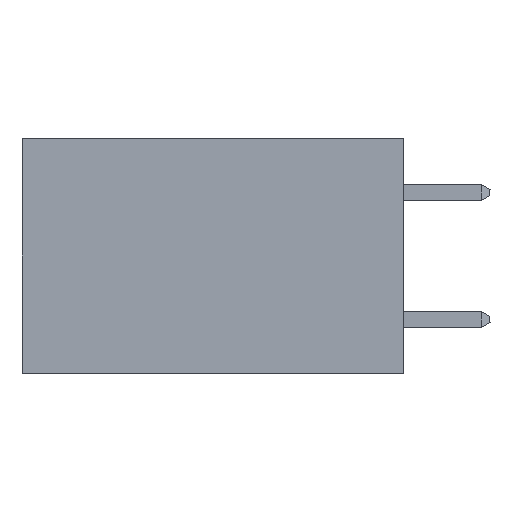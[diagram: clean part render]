
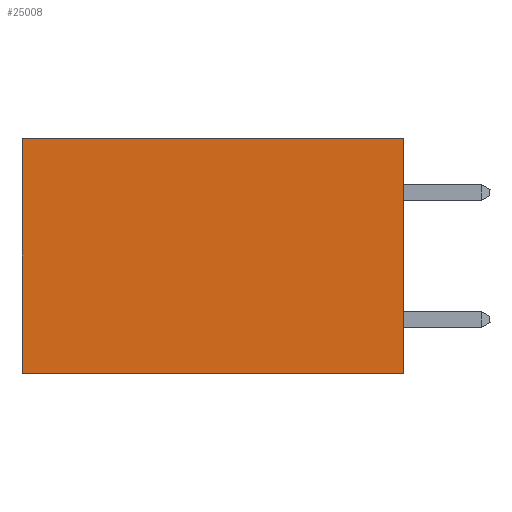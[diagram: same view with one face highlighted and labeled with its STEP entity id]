
A CAD part, left-side view. The second image highlights one B-rep face of the part: STEP entity #25008.
In plain terms, the highlighted planar face has unit normal (-1, 0, 0).
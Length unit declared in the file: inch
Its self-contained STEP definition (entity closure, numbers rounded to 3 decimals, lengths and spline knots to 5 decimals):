
#365 = VECTOR ( 'NONE', #31459, 39.37008 ) ;
#2578 = CARTESIAN_POINT ( 'NONE',  ( 0.2875, 0., -0.37 ) ) ;
#3232 = VERTEX_POINT ( 'NONE', #40267 ) ;
#3275 = ORIENTED_EDGE ( 'NONE', *, *, #23552, .F. ) ;
#4162 = CARTESIAN_POINT ( 'NONE',  ( 0.2875, 0., 0. ) ) ;
#5787 = DIRECTION ( 'NONE',  ( 0., 1., 0. ) ) ;
#5964 = PLANE ( 'NONE',  #34227 ) ;
#6248 = DIRECTION ( 'NONE',  ( 0., 0., -1. ) ) ;
#8060 = FACE_OUTER_BOUND ( 'NONE', #42667, .T. ) ;
#8094 = CARTESIAN_POINT ( 'NONE',  ( 0.2875, 0., 0. ) ) ;
#10351 = VECTOR ( 'NONE', #23497, 39.37008 ) ;
#11244 = VECTOR ( 'NONE', #5787, 39.37008 ) ;
#11322 = VECTOR ( 'NONE', #15116, 39.37008 ) ;
#13594 = ORIENTED_EDGE ( 'NONE', *, *, #41556, .T. ) ;
#15116 = DIRECTION ( 'NONE',  ( 0., 0., -1. ) ) ;
#15255 = VERTEX_POINT ( 'NONE', #42517 ) ;
#17210 = EDGE_CURVE ( 'NONE', #23805, #15255, #20139, .T. ) ;
#20139 = LINE ( 'NONE', #8094, #11322 ) ;
#22127 = CARTESIAN_POINT ( 'NONE',  ( 0.2875, 0.6, -0.37 ) ) ;
#23497 = DIRECTION ( 'NONE',  ( 0., 1., 0. ) ) ;
#23552 = EDGE_CURVE ( 'NONE', #15255, #36926, #37277, .T. ) ;
#23716 = LINE ( 'NONE', #34952, #365 ) ;
#23805 = VERTEX_POINT ( 'NONE', #4162 ) ;
#23999 = ORIENTED_EDGE ( 'NONE', *, *, #31661, .T. ) ;
#25008 = ADVANCED_FACE ( 'NONE', ( #8060 ), #5964, .F. ) ;
#27009 = LINE ( 'NONE', #40704, #10351 ) ;
#31459 = DIRECTION ( 'NONE',  ( 0., 0., -1. ) ) ;
#31661 = EDGE_CURVE ( 'NONE', #23805, #3232, #27009, .T. ) ;
#34227 = AXIS2_PLACEMENT_3D ( 'NONE', #36443, #39380, #6248 ) ;
#34595 = ORIENTED_EDGE ( 'NONE', *, *, #17210, .F. ) ;
#34952 = CARTESIAN_POINT ( 'NONE',  ( 0.2875, 0.6, 0. ) ) ;
#36443 = CARTESIAN_POINT ( 'NONE',  ( 0.2875, 0., 0. ) ) ;
#36926 = VERTEX_POINT ( 'NONE', #22127 ) ;
#37277 = LINE ( 'NONE', #2578, #11244 ) ;
#39380 = DIRECTION ( 'NONE',  ( 1., 0., 0. ) ) ;
#40267 = CARTESIAN_POINT ( 'NONE',  ( 0.2875, 0.6, 0. ) ) ;
#40704 = CARTESIAN_POINT ( 'NONE',  ( 0.2875, 0., 0. ) ) ;
#41556 = EDGE_CURVE ( 'NONE', #3232, #36926, #23716, .T. ) ;
#42517 = CARTESIAN_POINT ( 'NONE',  ( 0.2875, 0., -0.37 ) ) ;
#42667 = EDGE_LOOP ( 'NONE', ( #13594, #3275, #34595, #23999 ) ) ;
